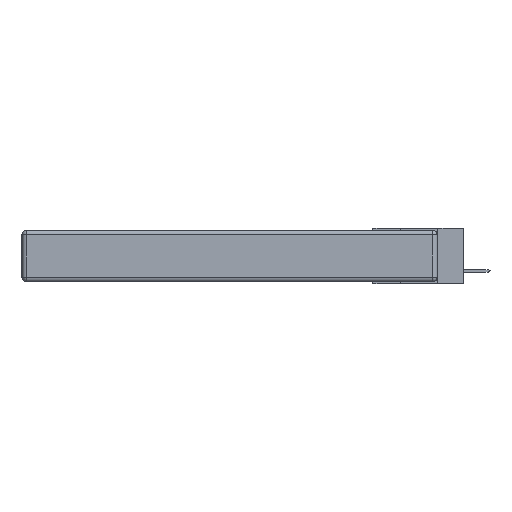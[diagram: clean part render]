
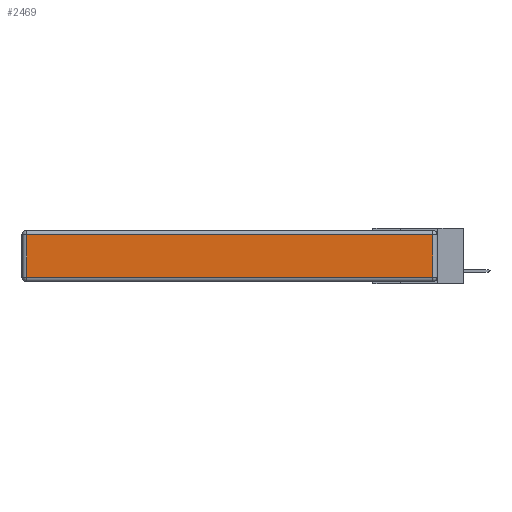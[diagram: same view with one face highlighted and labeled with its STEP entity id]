
A CAD part, left-side view. The second image highlights one B-rep face of the part: STEP entity #2469.
In plain terms, the highlighted planar face has unit normal (-1, 0, 0).
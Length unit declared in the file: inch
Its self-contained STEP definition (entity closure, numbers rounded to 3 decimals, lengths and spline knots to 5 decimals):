
#211 = DIRECTION ( 'NONE',  ( -1., 0., 0. ) ) ;
#1255 = CARTESIAN_POINT ( 'NONE',  ( 0., 0.03, -0.313 ) ) ;
#1362 = AXIS2_PLACEMENT_3D ( 'NONE', #23473, #211, #25616 ) ;
#1643 = DIRECTION ( 'NONE',  ( 0., 0., -1. ) ) ;
#2469 = ADVANCED_FACE ( 'NONE', ( #24029 ), #8686, .T. ) ;
#3320 = DIRECTION ( 'NONE',  ( 0., -1., 0. ) ) ;
#3494 = ORIENTED_EDGE ( 'NONE', *, *, #25569, .T. ) ;
#3560 = DIRECTION ( 'NONE',  ( 0., 0., 1. ) ) ;
#5057 = CARTESIAN_POINT ( 'NONE',  ( 0., 2.72, -0.313 ) ) ;
#5517 = VECTOR ( 'NONE', #3320, 39.37008 ) ;
#5543 = DIRECTION ( 'NONE',  ( 0., 1., 0. ) ) ;
#8254 = EDGE_CURVE ( 'NONE', #14324, #26556, #21682, .T. ) ;
#8279 = VECTOR ( 'NONE', #3560, 39.37008 ) ;
#8686 = PLANE ( 'NONE',  #1362 ) ;
#9842 = CARTESIAN_POINT ( 'NONE',  ( 0., 0., -0.313 ) ) ;
#10270 = ORIENTED_EDGE ( 'NONE', *, *, #8254, .T. ) ;
#10291 = LINE ( 'NONE', #18152, #17915 ) ;
#10693 = CARTESIAN_POINT ( 'NONE',  ( 0., 2.72, -0.03 ) ) ;
#12448 = CARTESIAN_POINT ( 'NONE',  ( 0., 0.03, -0.03 ) ) ;
#14324 = VERTEX_POINT ( 'NONE', #1255 ) ;
#14636 = VERTEX_POINT ( 'NONE', #5057 ) ;
#14815 = ORIENTED_EDGE ( 'NONE', *, *, #25131, .T. ) ;
#14929 = VERTEX_POINT ( 'NONE', #10693 ) ;
#15928 = VECTOR ( 'NONE', #1643, 39.37008 ) ;
#16672 = EDGE_CURVE ( 'NONE', #14636, #14324, #17758, .T. ) ;
#17758 = LINE ( 'NONE', #9842, #5517 ) ;
#17915 = VECTOR ( 'NONE', #5543, 39.37008 ) ;
#18152 = CARTESIAN_POINT ( 'NONE',  ( 0., 2.75, -0.03 ) ) ;
#18659 = EDGE_LOOP ( 'NONE', ( #26532, #10270, #3494, #14815 ) ) ;
#18704 = CARTESIAN_POINT ( 'NONE',  ( 0., 0.03, -0.343 ) ) ;
#19581 = LINE ( 'NONE', #24760, #15928 ) ;
#21682 = LINE ( 'NONE', #18704, #8279 ) ;
#23473 = CARTESIAN_POINT ( 'NONE',  ( 0., 0., -0.343 ) ) ;
#24029 = FACE_OUTER_BOUND ( 'NONE', #18659, .T. ) ;
#24760 = CARTESIAN_POINT ( 'NONE',  ( 0., 2.72, -0.343 ) ) ;
#25131 = EDGE_CURVE ( 'NONE', #14929, #14636, #19581, .T. ) ;
#25569 = EDGE_CURVE ( 'NONE', #26556, #14929, #10291, .T. ) ;
#25616 = DIRECTION ( 'NONE',  ( 0., 0., 1. ) ) ;
#26532 = ORIENTED_EDGE ( 'NONE', *, *, #16672, .T. ) ;
#26556 = VERTEX_POINT ( 'NONE', #12448 ) ;
